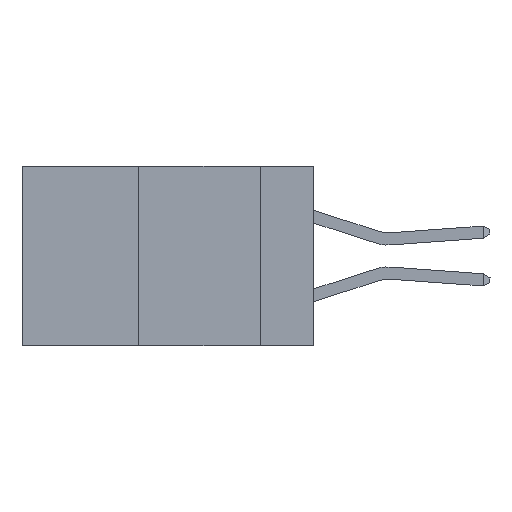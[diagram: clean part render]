
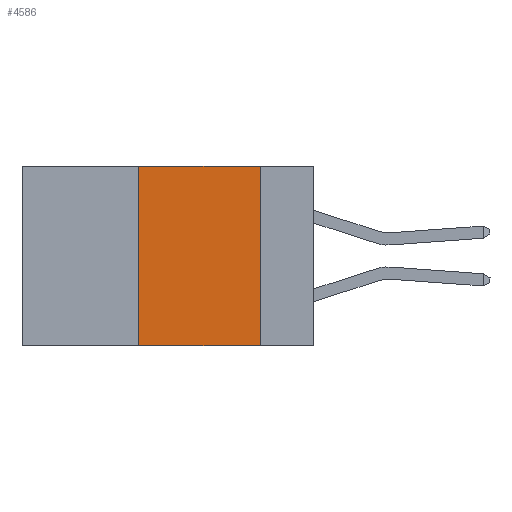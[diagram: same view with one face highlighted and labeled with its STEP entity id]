
A CAD part, left-side view. The second image highlights one B-rep face of the part: STEP entity #4586.
In plain terms, the highlighted planar face has unit normal (-1, 0, 0).
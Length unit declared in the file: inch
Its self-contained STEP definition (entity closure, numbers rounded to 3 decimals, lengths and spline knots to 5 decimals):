
#304 = CARTESIAN_POINT ( 'NONE',  ( 0., 0.6, 0. ) ) ;
#582 = EDGE_CURVE ( 'NONE', #7585, #19893, #4064, .T. ) ;
#865 = CARTESIAN_POINT ( 'NONE',  ( 0., 0.11, 0. ) ) ;
#2672 = AXIS2_PLACEMENT_3D ( 'NONE', #13999, #17369, #7479 ) ;
#3319 = ORIENTED_EDGE ( 'NONE', *, *, #14508, .F. ) ;
#4064 = LINE ( 'NONE', #304, #12364 ) ;
#4586 = ADVANCED_FACE ( 'NONE', ( #8775 ), #5791, .F. ) ;
#5281 = CARTESIAN_POINT ( 'NONE',  ( 0., 0.36, 0. ) ) ;
#5426 = CARTESIAN_POINT ( 'NONE',  ( 0., 0.6, -0.37 ) ) ;
#5791 = PLANE ( 'NONE',  #2672 ) ;
#6945 = ORIENTED_EDGE ( 'NONE', *, *, #16348, .T. ) ;
#7479 = DIRECTION ( 'NONE',  ( 0., 0., -1. ) ) ;
#7585 = VERTEX_POINT ( 'NONE', #10566 ) ;
#8264 = VECTOR ( 'NONE', #10435, 39.37008 ) ;
#8775 = FACE_OUTER_BOUND ( 'NONE', #10459, .T. ) ;
#10435 = DIRECTION ( 'NONE',  ( 0., -1., 0. ) ) ;
#10459 = EDGE_LOOP ( 'NONE', ( #12951, #16097, #3319, #6945 ) ) ;
#10566 = CARTESIAN_POINT ( 'NONE',  ( 0., 0.36, 0. ) ) ;
#11488 = VECTOR ( 'NONE', #20580, 39.37008 ) ;
#11912 = DIRECTION ( 'NONE',  ( 0., -1., 0. ) ) ;
#12364 = VECTOR ( 'NONE', #11912, 39.37008 ) ;
#12861 = EDGE_CURVE ( 'NONE', #19893, #18781, #15819, .T. ) ;
#12951 = ORIENTED_EDGE ( 'NONE', *, *, #12861, .F. ) ;
#13001 = VERTEX_POINT ( 'NONE', #17705 ) ;
#13999 = CARTESIAN_POINT ( 'NONE',  ( 0., 0.6, 0. ) ) ;
#14433 = VECTOR ( 'NONE', #15173, 39.37008 ) ;
#14508 = EDGE_CURVE ( 'NONE', #13001, #7585, #17857, .T. ) ;
#15173 = DIRECTION ( 'NONE',  ( 0., 0., 1. ) ) ;
#15819 = LINE ( 'NONE', #18993, #11488 ) ;
#16097 = ORIENTED_EDGE ( 'NONE', *, *, #582, .F. ) ;
#16348 = EDGE_CURVE ( 'NONE', #13001, #18781, #17009, .T. ) ;
#17009 = LINE ( 'NONE', #5426, #8264 ) ;
#17369 = DIRECTION ( 'NONE',  ( 1., 0., 0. ) ) ;
#17705 = CARTESIAN_POINT ( 'NONE',  ( 0., 0.36, -0.37 ) ) ;
#17857 = LINE ( 'NONE', #5281, #14433 ) ;
#18781 = VERTEX_POINT ( 'NONE', #21031 ) ;
#18993 = CARTESIAN_POINT ( 'NONE',  ( 0., 0.11, 0. ) ) ;
#19893 = VERTEX_POINT ( 'NONE', #865 ) ;
#20580 = DIRECTION ( 'NONE',  ( 0., 0., -1. ) ) ;
#21031 = CARTESIAN_POINT ( 'NONE',  ( 0., 0.11, -0.37 ) ) ;
